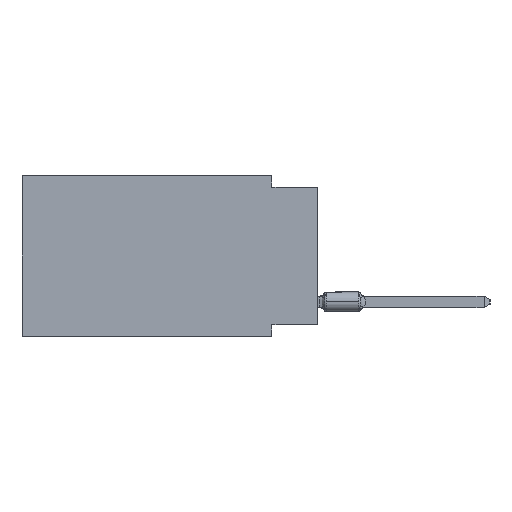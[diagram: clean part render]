
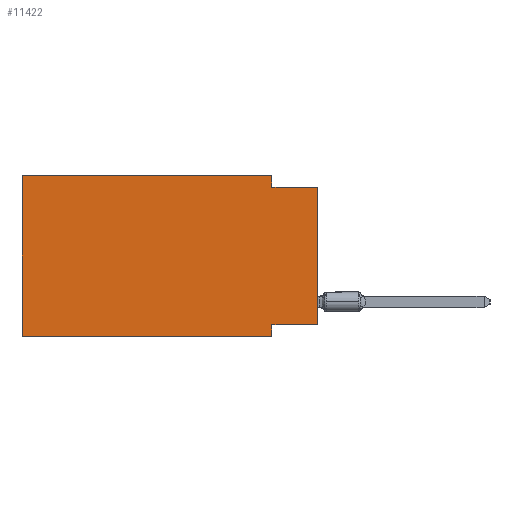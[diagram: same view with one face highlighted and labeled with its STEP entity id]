
A CAD part, left-side view. The second image highlights one B-rep face of the part: STEP entity #11422.
In plain terms, the highlighted planar face has unit normal (-1, 0, 0).
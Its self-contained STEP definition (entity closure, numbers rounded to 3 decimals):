
#328 = CARTESIAN_POINT ( 'NONE',  ( 0., 0., -0.635 ) ) ;
#448 = ORIENTED_EDGE ( 'NONE', *, *, #1059, .F. ) ;
#1059 = EDGE_CURVE ( 'NONE', #13280, #5328, #10703, .T. ) ;
#1131 = DIRECTION ( 'NONE',  ( 0., 0., -1. ) ) ;
#1430 = ORIENTED_EDGE ( 'NONE', *, *, #18996, .F. ) ;
#1779 = LINE ( 'NONE', #9274, #16181 ) ;
#2581 = DIRECTION ( 'NONE',  ( 0., 0., 1. ) ) ;
#3780 = CARTESIAN_POINT ( 'NONE',  ( 0., 0., 0. ) ) ;
#4780 = CARTESIAN_POINT ( 'NONE',  ( 0., 2.54, -8.89 ) ) ;
#5328 = VERTEX_POINT ( 'NONE', #16597 ) ;
#5855 = CARTESIAN_POINT ( 'NONE',  ( 0., 2.54, -8.255 ) ) ;
#6470 = EDGE_LOOP ( 'NONE', ( #23589, #24205, #448, #10727, #1430, #16873, #18026, #13790 ) ) ;
#7174 = VERTEX_POINT ( 'NONE', #22167 ) ;
#7310 = AXIS2_PLACEMENT_3D ( 'NONE', #22454, #14985, #16705 ) ;
#7452 = DIRECTION ( 'NONE',  ( 0., 0., 1. ) ) ;
#7568 = LINE ( 'NONE', #3780, #13319 ) ;
#8572 = CARTESIAN_POINT ( 'NONE',  ( 0., 16.383, -8.89 ) ) ;
#8745 = CARTESIAN_POINT ( 'NONE',  ( 0., 2.54, 0. ) ) ;
#8815 = LINE ( 'NONE', #18263, #13754 ) ;
#8951 = DIRECTION ( 'NONE',  ( 0., 0., -1. ) ) ;
#9274 = CARTESIAN_POINT ( 'NONE',  ( 0., 0., -8.255 ) ) ;
#9821 = LINE ( 'NONE', #21465, #23074 ) ;
#10703 = LINE ( 'NONE', #8745, #13825 ) ;
#10727 = ORIENTED_EDGE ( 'NONE', *, *, #20806, .F. ) ;
#11422 = ADVANCED_FACE ( 'NONE', ( #18417 ), #22336, .F. ) ;
#11680 = EDGE_CURVE ( 'NONE', #5328, #15537, #19858, .T. ) ;
#12264 = DIRECTION ( 'NONE',  ( 0., -1., 0. ) ) ;
#12266 = VERTEX_POINT ( 'NONE', #16769 ) ;
#13280 = VERTEX_POINT ( 'NONE', #15434 ) ;
#13319 = VECTOR ( 'NONE', #7452, 1000. ) ;
#13754 = VECTOR ( 'NONE', #16554, 1000. ) ;
#13790 = ORIENTED_EDGE ( 'NONE', *, *, #22529, .F. ) ;
#13825 = VECTOR ( 'NONE', #1131, 1000. ) ;
#14610 = VECTOR ( 'NONE', #12264, 1000. ) ;
#14985 = DIRECTION ( 'NONE',  ( 1., 0., 0. ) ) ;
#15041 = DIRECTION ( 'NONE',  ( 0., 1., 0. ) ) ;
#15206 = EDGE_CURVE ( 'NONE', #15352, #16941, #23925, .T. ) ;
#15352 = VERTEX_POINT ( 'NONE', #5855 ) ;
#15434 = CARTESIAN_POINT ( 'NONE',  ( 0., 2.54, 0. ) ) ;
#15537 = VERTEX_POINT ( 'NONE', #328 ) ;
#16068 = DIRECTION ( 'NONE',  ( 0., -1., 0. ) ) ;
#16181 = VECTOR ( 'NONE', #15041, 1000. ) ;
#16410 = VERTEX_POINT ( 'NONE', #18936 ) ;
#16554 = DIRECTION ( 'NONE',  ( 0., -1., 0. ) ) ;
#16597 = CARTESIAN_POINT ( 'NONE',  ( 0., 2.54, -0.635 ) ) ;
#16705 = DIRECTION ( 'NONE',  ( 0., 0., -1. ) ) ;
#16769 = CARTESIAN_POINT ( 'NONE',  ( 0., 16.383, 0. ) ) ;
#16873 = ORIENTED_EDGE ( 'NONE', *, *, #22318, .T. ) ;
#16941 = VERTEX_POINT ( 'NONE', #23557 ) ;
#17202 = VECTOR ( 'NONE', #8951, 1000. ) ;
#18026 = ORIENTED_EDGE ( 'NONE', *, *, #15206, .F. ) ;
#18263 = CARTESIAN_POINT ( 'NONE',  ( 0., 16.383, 0. ) ) ;
#18417 = FACE_OUTER_BOUND ( 'NONE', #6470, .T. ) ;
#18936 = CARTESIAN_POINT ( 'NONE',  ( 0., 0., -8.255 ) ) ;
#18996 = EDGE_CURVE ( 'NONE', #7174, #12266, #9821, .T. ) ;
#19498 = CARTESIAN_POINT ( 'NONE',  ( 0., 0., -0.635 ) ) ;
#19858 = LINE ( 'NONE', #19498, #23372 ) ;
#20806 = EDGE_CURVE ( 'NONE', #12266, #13280, #8815, .T. ) ;
#20934 = EDGE_CURVE ( 'NONE', #16410, #15537, #7568, .T. ) ;
#21105 = LINE ( 'NONE', #8572, #14610 ) ;
#21465 = CARTESIAN_POINT ( 'NONE',  ( 0., 16.383, 0. ) ) ;
#22167 = CARTESIAN_POINT ( 'NONE',  ( 0., 16.383, -8.89 ) ) ;
#22318 = EDGE_CURVE ( 'NONE', #7174, #16941, #21105, .T. ) ;
#22336 = PLANE ( 'NONE',  #7310 ) ;
#22454 = CARTESIAN_POINT ( 'NONE',  ( 0., 16.383, 0. ) ) ;
#22529 = EDGE_CURVE ( 'NONE', #16410, #15352, #1779, .T. ) ;
#23074 = VECTOR ( 'NONE', #2581, 1000. ) ;
#23372 = VECTOR ( 'NONE', #16068, 1000. ) ;
#23557 = CARTESIAN_POINT ( 'NONE',  ( 0., 2.54, -8.89 ) ) ;
#23589 = ORIENTED_EDGE ( 'NONE', *, *, #20934, .T. ) ;
#23925 = LINE ( 'NONE', #4780, #17202 ) ;
#24205 = ORIENTED_EDGE ( 'NONE', *, *, #11680, .F. ) ;
